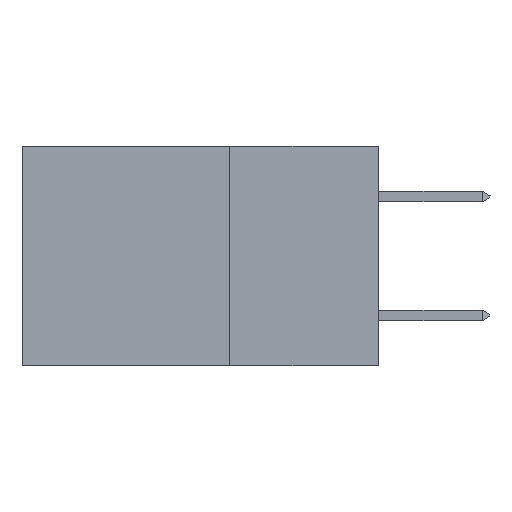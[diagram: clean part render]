
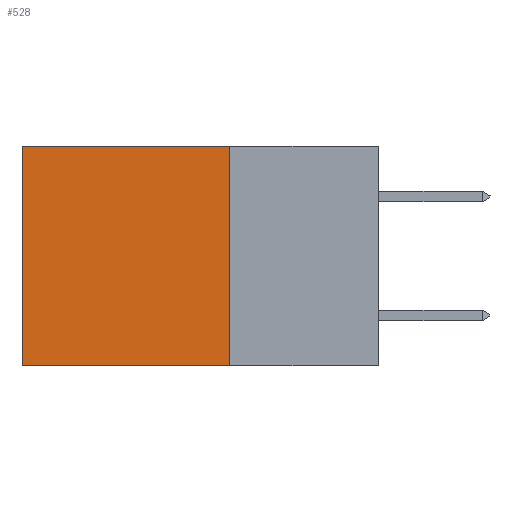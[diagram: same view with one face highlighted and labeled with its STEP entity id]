
A CAD part, left-side view. The second image highlights one B-rep face of the part: STEP entity #528.
In plain terms, the highlighted planar face has unit normal (-1, 0, 0).
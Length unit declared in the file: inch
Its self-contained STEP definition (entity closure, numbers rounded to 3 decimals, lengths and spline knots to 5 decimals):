
#391 = ORIENTED_EDGE ( 'NONE', *, *, #5547, .F. ) ;
#417 = DIRECTION ( 'NONE',  ( 0., 0., -1. ) ) ;
#489 = ORIENTED_EDGE ( 'NONE', *, *, #12768, .T. ) ;
#528 = ADVANCED_FACE ( 'NONE', ( #15681 ), #18889, .F. ) ;
#595 = DIRECTION ( 'NONE',  ( 0., 1., 0. ) ) ;
#2648 = CARTESIAN_POINT ( 'NONE',  ( 0.2615, 0.25, -0.37 ) ) ;
#3170 = EDGE_CURVE ( 'NONE', #8476, #16101, #7463, .T. ) ;
#4259 = VECTOR ( 'NONE', #20325, 39.37008 ) ;
#4324 = CARTESIAN_POINT ( 'NONE',  ( 0.2615, 0.25, -0.37 ) ) ;
#5132 = LINE ( 'NONE', #11675, #16234 ) ;
#5489 = EDGE_CURVE ( 'NONE', #18430, #16101, #5132, .T. ) ;
#5547 = EDGE_CURVE ( 'NONE', #18692, #8476, #18816, .T. ) ;
#7463 = LINE ( 'NONE', #13887, #10688 ) ;
#8476 = VERTEX_POINT ( 'NONE', #4324 ) ;
#9083 = DIRECTION ( 'NONE',  ( 0., 1., 0. ) ) ;
#10688 = VECTOR ( 'NONE', #9083, 39.37008 ) ;
#10769 = CARTESIAN_POINT ( 'NONE',  ( 0.2615, 0.25, -0.37 ) ) ;
#11564 = LINE ( 'NONE', #16378, #16040 ) ;
#11675 = CARTESIAN_POINT ( 'NONE',  ( 0.2615, 0.6, -0.37 ) ) ;
#12768 = EDGE_CURVE ( 'NONE', #18692, #18430, #11564, .T. ) ;
#13887 = CARTESIAN_POINT ( 'NONE',  ( 0.2615, 0.25, -0.37 ) ) ;
#15681 = FACE_OUTER_BOUND ( 'NONE', #18070, .T. ) ;
#16040 = VECTOR ( 'NONE', #595, 39.37008 ) ;
#16101 = VERTEX_POINT ( 'NONE', #20407 ) ;
#16234 = VECTOR ( 'NONE', #417, 39.37008 ) ;
#16378 = CARTESIAN_POINT ( 'NONE',  ( 0.2615, 0.25, 0. ) ) ;
#17130 = CARTESIAN_POINT ( 'NONE',  ( 0.2615, 0.25, 0. ) ) ;
#17399 = DIRECTION ( 'NONE',  ( 1., 0., 0. ) ) ;
#17770 = AXIS2_PLACEMENT_3D ( 'NONE', #10769, #17399, #20714 ) ;
#18070 = EDGE_LOOP ( 'NONE', ( #19309, #19080, #391, #489 ) ) ;
#18430 = VERTEX_POINT ( 'NONE', #19495 ) ;
#18692 = VERTEX_POINT ( 'NONE', #17130 ) ;
#18816 = LINE ( 'NONE', #2648, #4259 ) ;
#18889 = PLANE ( 'NONE',  #17770 ) ;
#19080 = ORIENTED_EDGE ( 'NONE', *, *, #3170, .F. ) ;
#19309 = ORIENTED_EDGE ( 'NONE', *, *, #5489, .T. ) ;
#19495 = CARTESIAN_POINT ( 'NONE',  ( 0.2615, 0.6, 0. ) ) ;
#20325 = DIRECTION ( 'NONE',  ( 0., 0., -1. ) ) ;
#20407 = CARTESIAN_POINT ( 'NONE',  ( 0.2615, 0.6, -0.37 ) ) ;
#20714 = DIRECTION ( 'NONE',  ( 0., 0., -1. ) ) ;
